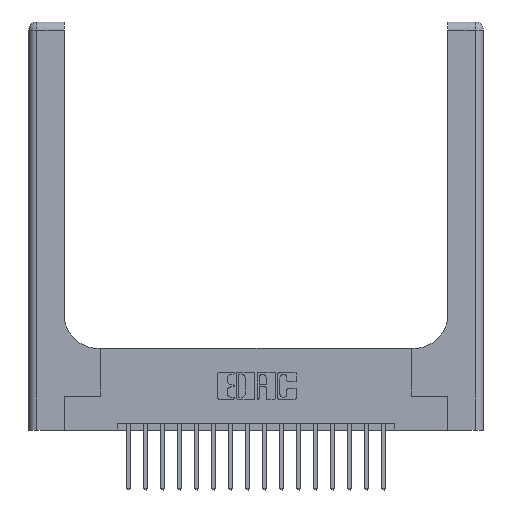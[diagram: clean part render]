
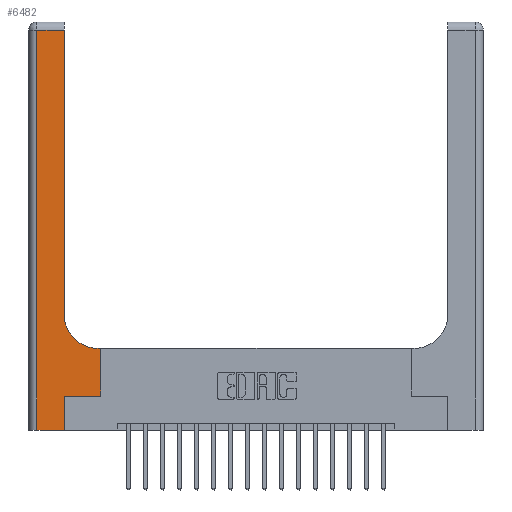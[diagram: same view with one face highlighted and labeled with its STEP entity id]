
A CAD part, top view. The second image highlights one B-rep face of the part: STEP entity #6482.
In plain terms, the highlighted planar face has unit normal (0, 0, 1).
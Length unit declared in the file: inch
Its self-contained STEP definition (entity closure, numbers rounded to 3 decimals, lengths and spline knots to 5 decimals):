
#93 = CARTESIAN_POINT ( 'NONE',  ( 0., 2.94, 0.37 ) ) ;
#212 = DIRECTION ( 'NONE',  ( 1., 0., 0. ) ) ;
#331 = CARTESIAN_POINT ( 'NONE',  ( 0.528, 0.6, 0.37 ) ) ;
#646 = CARTESIAN_POINT ( 'NONE',  ( 0.06, 3., 0.37 ) ) ;
#814 = ORIENTED_EDGE ( 'NONE', *, *, #10001, .T. ) ;
#1125 = LINE ( 'NONE', #4008, #12322 ) ;
#1492 = LINE ( 'NONE', #12507, #4337 ) ;
#1671 = DIRECTION ( 'NONE',  ( 1., 0., 0. ) ) ;
#1714 = DIRECTION ( 'NONE',  ( -1., 0., 0. ) ) ;
#1911 = ORIENTED_EDGE ( 'NONE', *, *, #14628, .T. ) ;
#2186 = ORIENTED_EDGE ( 'NONE', *, *, #4464, .T. ) ;
#2338 = ORIENTED_EDGE ( 'NONE', *, *, #19431, .T. ) ;
#2763 = ORIENTED_EDGE ( 'NONE', *, *, #3600, .T. ) ;
#3600 = EDGE_CURVE ( 'NONE', #15207, #7541, #3797, .T. ) ;
#3797 = LINE ( 'NONE', #9858, #6567 ) ;
#3828 = VERTEX_POINT ( 'NONE', #331 ) ;
#4008 = CARTESIAN_POINT ( 'NONE',  ( 0.26, 0.6, 0.37 ) ) ;
#4087 = VECTOR ( 'NONE', #8382, 39.37008 ) ;
#4337 = VECTOR ( 'NONE', #212, 39.37008 ) ;
#4365 = CARTESIAN_POINT ( 'NONE',  ( 0.26, 0.85, 0.37 ) ) ;
#4464 = EDGE_CURVE ( 'NONE', #13120, #15207, #5720, .T. ) ;
#4924 = ORIENTED_EDGE ( 'NONE', *, *, #16664, .T. ) ;
#5711 = DIRECTION ( 'NONE',  ( -1., 0., 0. ) ) ;
#5720 = LINE ( 'NONE', #15727, #17345 ) ;
#5882 = CARTESIAN_POINT ( 'NONE',  ( 0., 3., 0.37 ) ) ;
#6482 = ADVANCED_FACE ( 'NONE', ( #10345 ), #16562, .F. ) ;
#6567 = VECTOR ( 'NONE', #9949, 39.37008 ) ;
#6618 = CARTESIAN_POINT ( 'NONE',  ( 0.528, 0.25, 0.37 ) ) ;
#7160 = VECTOR ( 'NONE', #16192, 39.37008 ) ;
#7279 = EDGE_LOOP ( 'NONE', ( #1911, #12190, #814, #8397, #2186, #2763, #4924, #2338, #7960 ) ) ;
#7406 = CARTESIAN_POINT ( 'NONE',  ( 0.51, 0.6, 0.37 ) ) ;
#7541 = VERTEX_POINT ( 'NONE', #6618 ) ;
#7960 = ORIENTED_EDGE ( 'NONE', *, *, #12411, .T. ) ;
#8382 = DIRECTION ( 'NONE',  ( 0., -1., 0. ) ) ;
#8397 = ORIENTED_EDGE ( 'NONE', *, *, #18222, .T. ) ;
#8788 = DIRECTION ( 'NONE',  ( 0., 1., 0. ) ) ;
#9132 = VERTEX_POINT ( 'NONE', #19389 ) ;
#9204 = VERTEX_POINT ( 'NONE', #7406 ) ;
#9346 = VERTEX_POINT ( 'NONE', #18214 ) ;
#9447 = AXIS2_PLACEMENT_3D ( 'NONE', #14947, #12393, #1671 ) ;
#9527 = DIRECTION ( 'NONE',  ( -1., 0., 0. ) ) ;
#9858 = CARTESIAN_POINT ( 'NONE',  ( 0.265, 0.25, 0.37 ) ) ;
#9949 = DIRECTION ( 'NONE',  ( 1., 0., 0. ) ) ;
#10001 = EDGE_CURVE ( 'NONE', #18704, #9346, #12938, .T. ) ;
#10332 = LINE ( 'NONE', #19537, #18355 ) ;
#10345 = FACE_OUTER_BOUND ( 'NONE', #7279, .T. ) ;
#10595 = CARTESIAN_POINT ( 'NONE',  ( 0.06, 2.94, 0.37 ) ) ;
#11564 = CARTESIAN_POINT ( 'NONE',  ( 0.528, 0.25, 0.37 ) ) ;
#11576 = VECTOR ( 'NONE', #9527, 39.37008 ) ;
#11652 = CARTESIAN_POINT ( 'NONE',  ( 0.265, 0., 0.37 ) ) ;
#11731 = DIRECTION ( 'NONE',  ( 0., 1., 0. ) ) ;
#12190 = ORIENTED_EDGE ( 'NONE', *, *, #16084, .T. ) ;
#12296 = CIRCLE ( 'NONE', #9447, 0.25 ) ;
#12322 = VECTOR ( 'NONE', #5711, 39.37008 ) ;
#12393 = DIRECTION ( 'NONE',  ( 0., 0., -1. ) ) ;
#12411 = EDGE_CURVE ( 'NONE', #9204, #18169, #12296, .T. ) ;
#12507 = CARTESIAN_POINT ( 'NONE',  ( 0., 0., 0.37 ) ) ;
#12938 = LINE ( 'NONE', #646, #4087 ) ;
#13120 = VERTEX_POINT ( 'NONE', #11652 ) ;
#13580 = LINE ( 'NONE', #93, #11576 ) ;
#14628 = EDGE_CURVE ( 'NONE', #18169, #9132, #10332, .T. ) ;
#14715 = LINE ( 'NONE', #11564, #7160 ) ;
#14807 = CARTESIAN_POINT ( 'NONE',  ( 0.265, 0.25, 0.37 ) ) ;
#14827 = AXIS2_PLACEMENT_3D ( 'NONE', #5882, #19553, #1714 ) ;
#14947 = CARTESIAN_POINT ( 'NONE',  ( 0.51, 0.85, 0.37 ) ) ;
#15207 = VERTEX_POINT ( 'NONE', #14807 ) ;
#15727 = CARTESIAN_POINT ( 'NONE',  ( 0.265, 0., 0.37 ) ) ;
#16084 = EDGE_CURVE ( 'NONE', #9132, #18704, #13580, .T. ) ;
#16192 = DIRECTION ( 'NONE',  ( 0., 1., 0. ) ) ;
#16562 = PLANE ( 'NONE',  #14827 ) ;
#16664 = EDGE_CURVE ( 'NONE', #7541, #3828, #14715, .T. ) ;
#17345 = VECTOR ( 'NONE', #8788, 39.37008 ) ;
#18169 = VERTEX_POINT ( 'NONE', #4365 ) ;
#18214 = CARTESIAN_POINT ( 'NONE',  ( 0.06, 0., 0.37 ) ) ;
#18222 = EDGE_CURVE ( 'NONE', #9346, #13120, #1492, .T. ) ;
#18355 = VECTOR ( 'NONE', #11731, 39.37008 ) ;
#18704 = VERTEX_POINT ( 'NONE', #10595 ) ;
#19389 = CARTESIAN_POINT ( 'NONE',  ( 0.26, 2.94, 0.37 ) ) ;
#19431 = EDGE_CURVE ( 'NONE', #3828, #9204, #1125, .T. ) ;
#19537 = CARTESIAN_POINT ( 'NONE',  ( 0.26, 3., 0.37 ) ) ;
#19553 = DIRECTION ( 'NONE',  ( 0., 0., -1. ) ) ;
